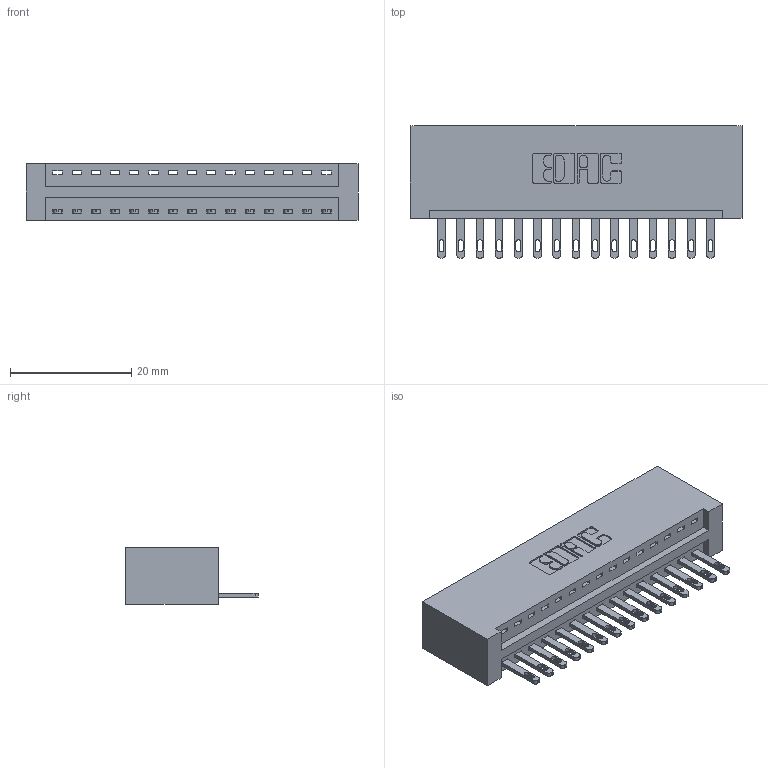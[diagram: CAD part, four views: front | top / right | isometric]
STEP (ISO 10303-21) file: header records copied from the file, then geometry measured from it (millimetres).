
FILE_DESCRIPTION (( 'STEP AP203' ), '1' );
FILE_NAME ('346-015-500-101.STEP', '2022-05-05T07:18:11', ( '' ), ( '' ), 'SwSTEP 2.0', 'SolidWorks 2020', '' );
FILE_SCHEMA (( 'CONFIG_CONTROL_DESIGN' ));
Length unit declared in the file: inch
Products named in the file (3): 345-292-001_345-293-100; 346 Part_No Mounting Lugs; 346-015-500-101
Assembly tree (16 placements, depth 2):
  346-015-500-101
    346 Part_No Mounting Lugs
    345-292-001_345-293-100  x15
Bounding box: 54.86 x 21.84 x 9.4 mm (x, y, z)
Volume: 5624.4 mm3; surface area: 6848.4 mm2
Topology: 16 solids, 16 shells, 924 faces, 2825 edges, 1882 vertices
Faces by surface type: plane 582, cylinder 342
Entity records: 12597 total; most frequent: CARTESIAN_POINT 2173, ORIENTED_EDGE 2122, DIRECTION 1947, EDGE_CURVE 1061, LINE 873, VECTOR 873, VERTEX_POINT 706, AXIS2_PLACEMENT_3D 537
